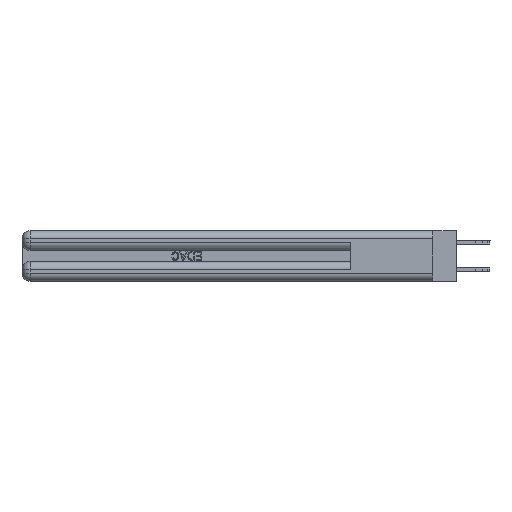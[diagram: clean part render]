
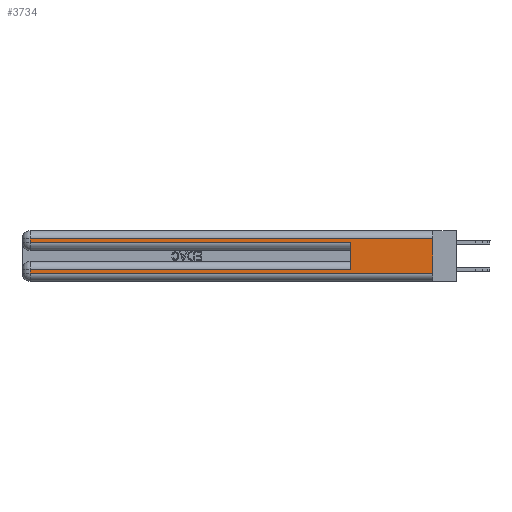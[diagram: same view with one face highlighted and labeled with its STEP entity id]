
A CAD part, left-side view. The second image highlights one B-rep face of the part: STEP entity #3734.
In plain terms, the highlighted planar face has unit normal (-1, 0, 0).
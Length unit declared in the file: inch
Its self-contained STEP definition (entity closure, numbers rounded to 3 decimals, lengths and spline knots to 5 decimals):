
#61 = CARTESIAN_POINT ( 'NONE',  ( 0., 2.94, 0.37 ) ) ;
#195 = EDGE_CURVE ( 'NONE', #7971, #34165, #30306, .T. ) ;
#233 = EDGE_CURVE ( 'NONE', #11068, #11421, #29271, .T. ) ;
#1757 = DIRECTION ( 'NONE',  ( 1., 0., 0. ) ) ;
#1853 = DIRECTION ( 'NONE',  ( 0., 1., 0. ) ) ;
#2179 = LINE ( 'NONE', #29580, #9531 ) ;
#2661 = CARTESIAN_POINT ( 'NONE',  ( 0., 0.6, 0.145 ) ) ;
#3734 = ADVANCED_FACE ( 'NONE', ( #4102 ), #11667, .F. ) ;
#4088 = ORIENTED_EDGE ( 'NONE', *, *, #7246, .F. ) ;
#4102 = FACE_OUTER_BOUND ( 'NONE', #32004, .T. ) ;
#5900 = LINE ( 'NONE', #14216, #34013 ) ;
#5935 = DIRECTION ( 'NONE',  ( 0., 0., -1. ) ) ;
#6370 = VERTEX_POINT ( 'NONE', #33748 ) ;
#7246 = EDGE_CURVE ( 'NONE', #11068, #34165, #37451, .T. ) ;
#7971 = VERTEX_POINT ( 'NONE', #13000 ) ;
#8639 = LINE ( 'NONE', #35731, #16031 ) ;
#9328 = ORIENTED_EDGE ( 'NONE', *, *, #233, .T. ) ;
#9390 = ORIENTED_EDGE ( 'NONE', *, *, #9608, .T. ) ;
#9531 = VECTOR ( 'NONE', #16504, 39.37008 ) ;
#9608 = EDGE_CURVE ( 'NONE', #11851, #6370, #8639, .T. ) ;
#10394 = DIRECTION ( 'NONE',  ( 0., 0., -1. ) ) ;
#10478 = EDGE_CURVE ( 'NONE', #24310, #6370, #2179, .T. ) ;
#11068 = VERTEX_POINT ( 'NONE', #27687 ) ;
#11421 = VERTEX_POINT ( 'NONE', #28441 ) ;
#11667 = PLANE ( 'NONE',  #39812 ) ;
#11851 = VERTEX_POINT ( 'NONE', #27685 ) ;
#13000 = CARTESIAN_POINT ( 'NONE',  ( 0., 2.94, 0.285 ) ) ;
#13714 = ORIENTED_EDGE ( 'NONE', *, *, #30175, .T. ) ;
#13851 = ORIENTED_EDGE ( 'NONE', *, *, #36272, .T. ) ;
#14216 = CARTESIAN_POINT ( 'NONE',  ( 0., 0., 0.31 ) ) ;
#16031 = VECTOR ( 'NONE', #16863, 39.37008 ) ;
#16504 = DIRECTION ( 'NONE',  ( 0., 0., -1. ) ) ;
#16863 = DIRECTION ( 'NONE',  ( 0., -1., 0. ) ) ;
#17399 = DIRECTION ( 'NONE',  ( 0., 1., 0. ) ) ;
#17549 = EDGE_CURVE ( 'NONE', #31663, #7971, #21344, .T. ) ;
#17629 = CARTESIAN_POINT ( 'NONE',  ( 0., 0., 0.37 ) ) ;
#17986 = CARTESIAN_POINT ( 'NONE',  ( 0., 2.94, 0.37 ) ) ;
#20812 = CARTESIAN_POINT ( 'NONE',  ( 0., 2.94, 0.31 ) ) ;
#20960 = VECTOR ( 'NONE', #1853, 39.37008 ) ;
#21037 = CARTESIAN_POINT ( 'NONE',  ( 0., 0., 0.31 ) ) ;
#21344 = LINE ( 'NONE', #17986, #34594 ) ;
#22237 = LINE ( 'NONE', #61, #34998 ) ;
#23817 = DIRECTION ( 'NONE',  ( 0., 0., -1. ) ) ;
#24052 = ORIENTED_EDGE ( 'NONE', *, *, #17549, .T. ) ;
#24310 = VERTEX_POINT ( 'NONE', #21037 ) ;
#26922 = CARTESIAN_POINT ( 'NONE',  ( 0., 0., 0.285 ) ) ;
#27348 = VECTOR ( 'NONE', #33093, 39.37008 ) ;
#27685 = CARTESIAN_POINT ( 'NONE',  ( 0., 2.94, 0.06 ) ) ;
#27687 = CARTESIAN_POINT ( 'NONE',  ( 0., 0.6, 0.085 ) ) ;
#28441 = CARTESIAN_POINT ( 'NONE',  ( 0., 2.94, 0.085 ) ) ;
#29271 = LINE ( 'NONE', #33367, #20960 ) ;
#29335 = ORIENTED_EDGE ( 'NONE', *, *, #10478, .F. ) ;
#29360 = ORIENTED_EDGE ( 'NONE', *, *, #195, .T. ) ;
#29541 = VECTOR ( 'NONE', #40812, 39.37008 ) ;
#29580 = CARTESIAN_POINT ( 'NONE',  ( 0., 0., 0.37 ) ) ;
#30175 = EDGE_CURVE ( 'NONE', #11421, #11851, #22237, .T. ) ;
#30262 = CARTESIAN_POINT ( 'NONE',  ( 0., 0.6, 0.285 ) ) ;
#30306 = LINE ( 'NONE', #26922, #27348 ) ;
#31663 = VERTEX_POINT ( 'NONE', #20812 ) ;
#32004 = EDGE_LOOP ( 'NONE', ( #29335, #13851, #24052, #29360, #4088, #9328, #13714, #9390 ) ) ;
#33093 = DIRECTION ( 'NONE',  ( 0., -1., 0. ) ) ;
#33367 = CARTESIAN_POINT ( 'NONE',  ( 0., 0., 0.085 ) ) ;
#33748 = CARTESIAN_POINT ( 'NONE',  ( 0., 0., 0.06 ) ) ;
#34013 = VECTOR ( 'NONE', #17399, 39.37008 ) ;
#34165 = VERTEX_POINT ( 'NONE', #30262 ) ;
#34594 = VECTOR ( 'NONE', #5935, 39.37008 ) ;
#34998 = VECTOR ( 'NONE', #10394, 39.37008 ) ;
#35731 = CARTESIAN_POINT ( 'NONE',  ( 0., 0., 0.06 ) ) ;
#36272 = EDGE_CURVE ( 'NONE', #24310, #31663, #5900, .T. ) ;
#37451 = LINE ( 'NONE', #2661, #29541 ) ;
#39812 = AXIS2_PLACEMENT_3D ( 'NONE', #17629, #1757, #23817 ) ;
#40812 = DIRECTION ( 'NONE',  ( 0., 0., 1. ) ) ;
